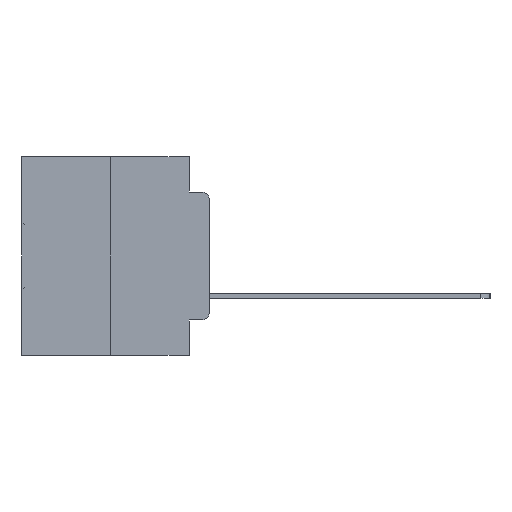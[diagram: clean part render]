
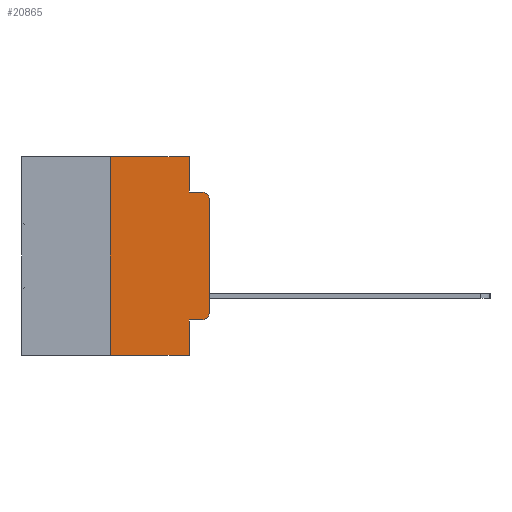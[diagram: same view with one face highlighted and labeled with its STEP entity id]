
A CAD part, left-side view. The second image highlights one B-rep face of the part: STEP entity #20865.
In plain terms, the highlighted planar face has unit normal (-1, 0, 0).
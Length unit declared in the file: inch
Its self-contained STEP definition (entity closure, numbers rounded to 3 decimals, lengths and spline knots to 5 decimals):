
#399 = ORIENTED_EDGE ( 'NONE', *, *, #9113, .F. ) ;
#750 = EDGE_CURVE ( 'NONE', #7592, #21777, #6424, .T. ) ;
#1857 = LINE ( 'NONE', #18309, #28220 ) ;
#2086 = EDGE_CURVE ( 'NONE', #11923, #14814, #30177, .T. ) ;
#2112 = CARTESIAN_POINT ( 'NONE',  ( 0., 0.051, -0.0885 ) ) ;
#2470 = ORIENTED_EDGE ( 'NONE', *, *, #15831, .T. ) ;
#2588 = PLANE ( 'NONE',  #12301 ) ;
#3200 = CARTESIAN_POINT ( 'NONE',  ( 0., 0.473, -0.5 ) ) ;
#4204 = AXIS2_PLACEMENT_3D ( 'NONE', #30063, #14913, #32563 ) ;
#4308 = VECTOR ( 'NONE', #6614, 39.37008 ) ;
#4855 = LINE ( 'NONE', #6255, #10930 ) ;
#4929 = CARTESIAN_POINT ( 'NONE',  ( 0., 0., -0.3915 ) ) ;
#4934 = ORIENTED_EDGE ( 'NONE', *, *, #12514, .F. ) ;
#5306 = CARTESIAN_POINT ( 'NONE',  ( 0., 0.02, -0.4115 ) ) ;
#5603 = EDGE_CURVE ( 'NONE', #9808, #11923, #14852, .T. ) ;
#5690 = VERTEX_POINT ( 'NONE', #22125 ) ;
#5943 = CARTESIAN_POINT ( 'NONE',  ( 0., 0., -0.1085 ) ) ;
#6255 = CARTESIAN_POINT ( 'NONE',  ( 0., 0., 0. ) ) ;
#6424 = LINE ( 'NONE', #3200, #32518 ) ;
#6577 = CARTESIAN_POINT ( 'NONE',  ( 0., 0.25, -0.5 ) ) ;
#6614 = DIRECTION ( 'NONE',  ( 0., -1., 0. ) ) ;
#6704 = VECTOR ( 'NONE', #20107, 39.37008 ) ;
#7380 = EDGE_CURVE ( 'NONE', #9808, #21777, #1857, .T. ) ;
#7592 = VERTEX_POINT ( 'NONE', #6577 ) ;
#7819 = ORIENTED_EDGE ( 'NONE', *, *, #19221, .T. ) ;
#8256 = DIRECTION ( 'NONE',  ( 0., -1., 0. ) ) ;
#9113 = EDGE_CURVE ( 'NONE', #7592, #16393, #9501, .T. ) ;
#9501 = LINE ( 'NONE', #23668, #28881 ) ;
#9808 = VERTEX_POINT ( 'NONE', #19454 ) ;
#10930 = VECTOR ( 'NONE', #26605, 39.37008 ) ;
#11417 = ORIENTED_EDGE ( 'NONE', *, *, #5603, .T. ) ;
#11923 = VERTEX_POINT ( 'NONE', #5306 ) ;
#12301 = AXIS2_PLACEMENT_3D ( 'NONE', #28019, #28122, #12984 ) ;
#12514 = EDGE_CURVE ( 'NONE', #5690, #21051, #26319, .T. ) ;
#12924 = DIRECTION ( 'NONE',  ( 0., 0., -1. ) ) ;
#12925 = AXIS2_PLACEMENT_3D ( 'NONE', #30377, #15226, #32861 ) ;
#12984 = DIRECTION ( 'NONE',  ( 0., 0., -1. ) ) ;
#13358 = EDGE_CURVE ( 'NONE', #16393, #5690, #31298, .T. ) ;
#13782 = ORIENTED_EDGE ( 'NONE', *, *, #2086, .T. ) ;
#14160 = EDGE_CURVE ( 'NONE', #21051, #24505, #26973, .T. ) ;
#14814 = VERTEX_POINT ( 'NONE', #4929 ) ;
#14852 = LINE ( 'NONE', #18632, #26783 ) ;
#14913 = DIRECTION ( 'NONE',  ( -1., 0., 0. ) ) ;
#14919 = CIRCLE ( 'NONE', #4204, 0.02 ) ;
#15182 = FACE_OUTER_BOUND ( 'NONE', #15824, .T. ) ;
#15226 = DIRECTION ( 'NONE',  ( -1., 0., 0. ) ) ;
#15307 = CARTESIAN_POINT ( 'NONE',  ( 0., 0.051, 0. ) ) ;
#15824 = EDGE_LOOP ( 'NONE', ( #7819, #2470, #16082, #4934, #25304, #399, #20871, #30748, #11417, #13782 ) ) ;
#15831 = EDGE_CURVE ( 'NONE', #23561, #24505, #14919, .T. ) ;
#15894 = DIRECTION ( 'NONE',  ( 0., 0., -1. ) ) ;
#16082 = ORIENTED_EDGE ( 'NONE', *, *, #14160, .F. ) ;
#16393 = VERTEX_POINT ( 'NONE', #25848 ) ;
#17286 = CARTESIAN_POINT ( 'NONE',  ( 0., 0.02, -0.0885 ) ) ;
#18309 = CARTESIAN_POINT ( 'NONE',  ( 0., 0.051, 0. ) ) ;
#18632 = CARTESIAN_POINT ( 'NONE',  ( 0., 0.051, -0.4115 ) ) ;
#18695 = VECTOR ( 'NONE', #12924, 39.37008 ) ;
#19221 = EDGE_CURVE ( 'NONE', #14814, #23561, #4855, .T. ) ;
#19234 = CARTESIAN_POINT ( 'NONE',  ( 0., 0.473, 0. ) ) ;
#19454 = CARTESIAN_POINT ( 'NONE',  ( 0., 0.051, -0.4115 ) ) ;
#20107 = DIRECTION ( 'NONE',  ( 0., -1., 0. ) ) ;
#20865 = ADVANCED_FACE ( 'NONE', ( #15182 ), #2588, .F. ) ;
#20871 = ORIENTED_EDGE ( 'NONE', *, *, #750, .T. ) ;
#21051 = VERTEX_POINT ( 'NONE', #23943 ) ;
#21205 = DIRECTION ( 'NONE',  ( 0., -1., 0. ) ) ;
#21777 = VERTEX_POINT ( 'NONE', #24461 ) ;
#22125 = CARTESIAN_POINT ( 'NONE',  ( 0., 0.051, 0. ) ) ;
#23561 = VERTEX_POINT ( 'NONE', #5943 ) ;
#23668 = CARTESIAN_POINT ( 'NONE',  ( 0., 0.25, 0. ) ) ;
#23943 = CARTESIAN_POINT ( 'NONE',  ( 0., 0.051, -0.0885 ) ) ;
#24461 = CARTESIAN_POINT ( 'NONE',  ( 0., 0.051, -0.5 ) ) ;
#24505 = VERTEX_POINT ( 'NONE', #17286 ) ;
#25304 = ORIENTED_EDGE ( 'NONE', *, *, #13358, .F. ) ;
#25848 = CARTESIAN_POINT ( 'NONE',  ( 0., 0.25, 0. ) ) ;
#26219 = DIRECTION ( 'NONE',  ( 0., 0., 1. ) ) ;
#26319 = LINE ( 'NONE', #15307, #18695 ) ;
#26605 = DIRECTION ( 'NONE',  ( 0., 0., 1. ) ) ;
#26783 = VECTOR ( 'NONE', #21205, 39.37008 ) ;
#26973 = LINE ( 'NONE', #2112, #6704 ) ;
#28019 = CARTESIAN_POINT ( 'NONE',  ( 0., 0.473, 0. ) ) ;
#28122 = DIRECTION ( 'NONE',  ( 1., 0., 0. ) ) ;
#28220 = VECTOR ( 'NONE', #15894, 39.37008 ) ;
#28881 = VECTOR ( 'NONE', #26219, 39.37008 ) ;
#30063 = CARTESIAN_POINT ( 'NONE',  ( 0., 0.02, -0.1085 ) ) ;
#30177 = CIRCLE ( 'NONE', #12925, 0.02 ) ;
#30377 = CARTESIAN_POINT ( 'NONE',  ( 0., 0.02, -0.3915 ) ) ;
#30748 = ORIENTED_EDGE ( 'NONE', *, *, #7380, .F. ) ;
#31298 = LINE ( 'NONE', #19234, #4308 ) ;
#32518 = VECTOR ( 'NONE', #8256, 39.37008 ) ;
#32563 = DIRECTION ( 'NONE',  ( 0., 0., -1. ) ) ;
#32861 = DIRECTION ( 'NONE',  ( 0., 0., -1. ) ) ;
